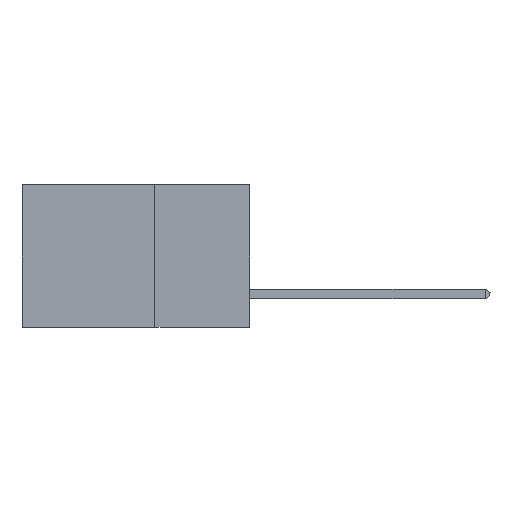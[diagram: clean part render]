
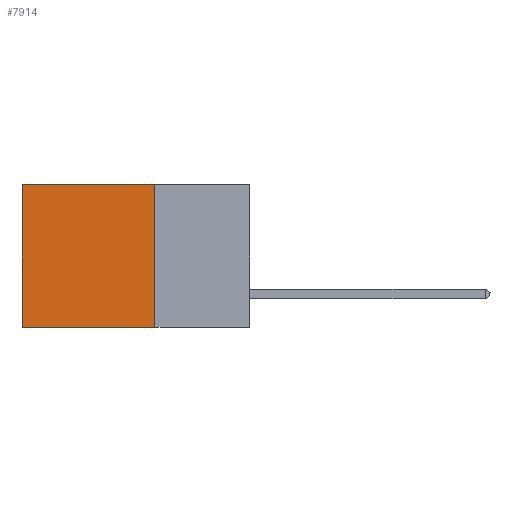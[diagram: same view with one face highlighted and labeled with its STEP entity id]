
A CAD part, left-side view. The second image highlights one B-rep face of the part: STEP entity #7914.
In plain terms, the highlighted planar face has unit normal (-1, 0, 0).
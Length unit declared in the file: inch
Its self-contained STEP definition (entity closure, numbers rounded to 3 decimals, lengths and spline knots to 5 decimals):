
#201 = VERTEX_POINT ( 'NONE', #9907 ) ;
#643 = LINE ( 'NONE', #4898, #12606 ) ;
#916 = VECTOR ( 'NONE', #6199, 39.37008 ) ;
#1183 = DIRECTION ( 'NONE',  ( 0., 0., -1. ) ) ;
#1711 = CARTESIAN_POINT ( 'NONE',  ( 0.2875, 0.6, 0. ) ) ;
#2687 = VERTEX_POINT ( 'NONE', #4079 ) ;
#3507 = ORIENTED_EDGE ( 'NONE', *, *, #11947, .F. ) ;
#3804 = ORIENTED_EDGE ( 'NONE', *, *, #12259, .T. ) ;
#4079 = CARTESIAN_POINT ( 'NONE',  ( 0.2875, 0.6, -0.375 ) ) ;
#4553 = ORIENTED_EDGE ( 'NONE', *, *, #7383, .F. ) ;
#4898 = CARTESIAN_POINT ( 'NONE',  ( 0.2875, 0.6, -0.375 ) ) ;
#4943 = DIRECTION ( 'NONE',  ( 0., 0., -1. ) ) ;
#5133 = VERTEX_POINT ( 'NONE', #6635 ) ;
#5423 = AXIS2_PLACEMENT_3D ( 'NONE', #10974, #11830, #4943 ) ;
#6168 = EDGE_LOOP ( 'NONE', ( #10919, #3507, #4553, #3804 ) ) ;
#6199 = DIRECTION ( 'NONE',  ( 0., 1., 0. ) ) ;
#6416 = LINE ( 'NONE', #9485, #10694 ) ;
#6635 = CARTESIAN_POINT ( 'NONE',  ( 0.2875, 0.25, 0. ) ) ;
#7203 = LINE ( 'NONE', #11291, #916 ) ;
#7383 = EDGE_CURVE ( 'NONE', #5133, #201, #10520, .T. ) ;
#7754 = PLANE ( 'NONE',  #5423 ) ;
#7914 = ADVANCED_FACE ( 'NONE', ( #8023 ), #7754, .F. ) ;
#8023 = FACE_OUTER_BOUND ( 'NONE', #6168, .T. ) ;
#8790 = DIRECTION ( 'NONE',  ( 0., 0., -1. ) ) ;
#9452 = CARTESIAN_POINT ( 'NONE',  ( 0.2875, 0.25, -0.375 ) ) ;
#9485 = CARTESIAN_POINT ( 'NONE',  ( 0.2875, 0.25, -0.375 ) ) ;
#9907 = CARTESIAN_POINT ( 'NONE',  ( 0.2875, 0.25, -0.375 ) ) ;
#10520 = LINE ( 'NONE', #9452, #10764 ) ;
#10694 = VECTOR ( 'NONE', #12693, 39.37008 ) ;
#10764 = VECTOR ( 'NONE', #1183, 39.37008 ) ;
#10919 = ORIENTED_EDGE ( 'NONE', *, *, #11166, .T. ) ;
#10974 = CARTESIAN_POINT ( 'NONE',  ( 0.2875, 0.25, -0.375 ) ) ;
#11113 = VERTEX_POINT ( 'NONE', #1711 ) ;
#11166 = EDGE_CURVE ( 'NONE', #11113, #2687, #643, .T. ) ;
#11291 = CARTESIAN_POINT ( 'NONE',  ( 0.2875, 0.25, 0. ) ) ;
#11830 = DIRECTION ( 'NONE',  ( 1., 0., 0. ) ) ;
#11947 = EDGE_CURVE ( 'NONE', #201, #2687, #6416, .T. ) ;
#12259 = EDGE_CURVE ( 'NONE', #5133, #11113, #7203, .T. ) ;
#12606 = VECTOR ( 'NONE', #8790, 39.37008 ) ;
#12693 = DIRECTION ( 'NONE',  ( 0., 1., 0. ) ) ;
